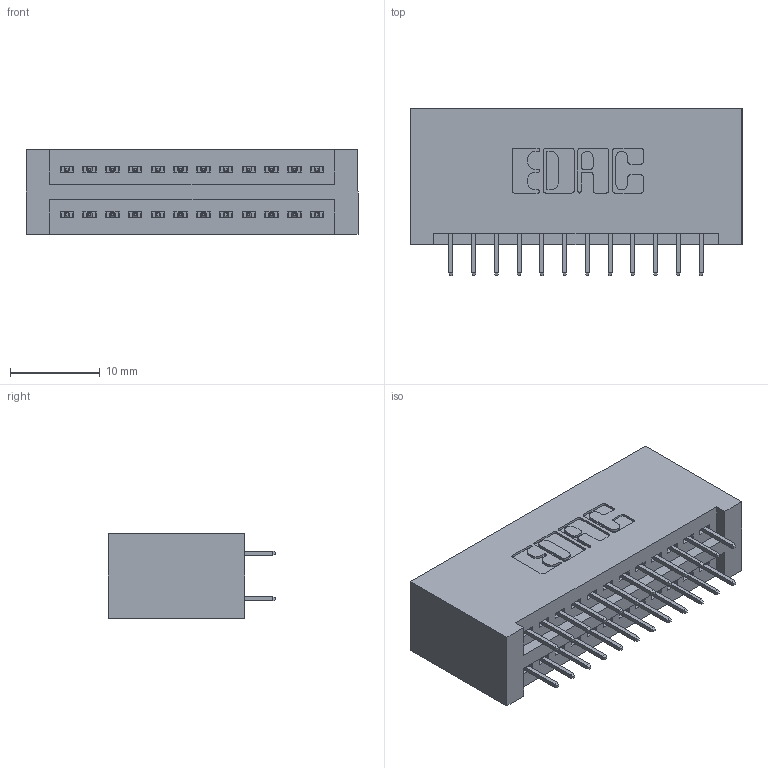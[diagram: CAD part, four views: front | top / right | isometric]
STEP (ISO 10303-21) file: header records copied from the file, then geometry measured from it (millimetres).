
FILE_DESCRIPTION (( 'STEP AP203' ), '1' );
FILE_NAME ('895-024-525-201.STEP', '2020-09-25T13:19:44', ( '' ), ( '' ), 'SwSTEP 2.0', 'SolidWorks 2020', '' );
FILE_SCHEMA (( 'CONFIG_CONTROL_DESIGN' ));
Length unit declared in the file: inch
Products named in the file (3): 345-292-001_345-293-125; 895-024-525-201; 845 Part_No Mounting Lugs
Assembly tree (25 placements, depth 2):
  895-024-525-201
    845 Part_No Mounting Lugs
    345-292-001_345-293-125  x24
Bounding box: 37.08 x 18.72 x 9.4 mm (x, y, z)
Volume: 3900.3 mm3; surface area: 5368.5 mm2
Topology: 25 solids, 25 shells, 1414 faces, 3989 edges, 2562 vertices
Faces by surface type: plane 1012, cylinder 402
Entity records: 13251 total; most frequent: CARTESIAN_POINT 2248, ORIENTED_EDGE 2182, DIRECTION 2015, EDGE_CURVE 1091, LINE 923, VECTOR 923, VERTEX_POINT 722, AXIS2_PLACEMENT_3D 546
